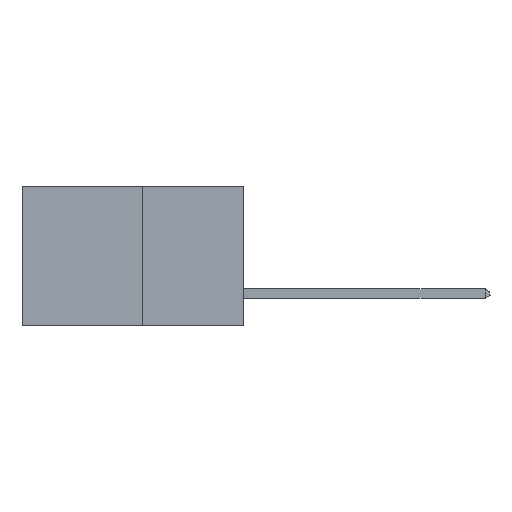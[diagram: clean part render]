
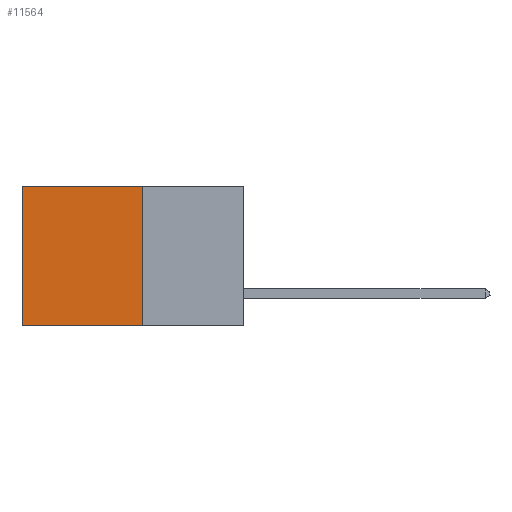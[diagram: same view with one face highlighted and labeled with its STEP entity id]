
A CAD part, left-side view. The second image highlights one B-rep face of the part: STEP entity #11564.
In plain terms, the highlighted planar face has unit normal (-1, 0, 0).
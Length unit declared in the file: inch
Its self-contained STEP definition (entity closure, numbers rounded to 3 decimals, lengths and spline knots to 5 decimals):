
#1414 = CARTESIAN_POINT ( 'NONE',  ( 0.277, 0.27, 0. ) ) ;
#2942 = DIRECTION ( 'NONE',  ( 0., 0., -1. ) ) ;
#2967 = CARTESIAN_POINT ( 'NONE',  ( 0.277, 0.27, -0.37 ) ) ;
#3269 = EDGE_CURVE ( 'NONE', #19605, #4331, #15075, .T. ) ;
#3989 = VECTOR ( 'NONE', #9598, 39.37008 ) ;
#4331 = VERTEX_POINT ( 'NONE', #9161 ) ;
#5077 = EDGE_LOOP ( 'NONE', ( #13645, #12473, #19442, #5239 ) ) ;
#5239 = ORIENTED_EDGE ( 'NONE', *, *, #6324, .T. ) ;
#5802 = VECTOR ( 'NONE', #19925, 39.37008 ) ;
#5838 = EDGE_CURVE ( 'NONE', #4331, #9906, #24892, .T. ) ;
#6324 = EDGE_CURVE ( 'NONE', #19605, #13140, #21268, .T. ) ;
#6867 = CARTESIAN_POINT ( 'NONE',  ( 0.277, 0.59, -0.37 ) ) ;
#7278 = CARTESIAN_POINT ( 'NONE',  ( 0.277, 0.27, -0.37 ) ) ;
#8807 = VECTOR ( 'NONE', #2942, 39.37008 ) ;
#9161 = CARTESIAN_POINT ( 'NONE',  ( 0.277, 0.27, -0.37 ) ) ;
#9311 = FACE_OUTER_BOUND ( 'NONE', #5077, .T. ) ;
#9427 = LINE ( 'NONE', #18610, #8807 ) ;
#9598 = DIRECTION ( 'NONE',  ( 0., 0., -1. ) ) ;
#9906 = VERTEX_POINT ( 'NONE', #6867 ) ;
#11564 = ADVANCED_FACE ( 'NONE', ( #9311 ), #13255, .F. ) ;
#11855 = AXIS2_PLACEMENT_3D ( 'NONE', #13756, #13218, #13209 ) ;
#12473 = ORIENTED_EDGE ( 'NONE', *, *, #5838, .F. ) ;
#13140 = VERTEX_POINT ( 'NONE', #23534 ) ;
#13209 = DIRECTION ( 'NONE',  ( 0., 0., -1. ) ) ;
#13218 = DIRECTION ( 'NONE',  ( 1., 0., 0. ) ) ;
#13255 = PLANE ( 'NONE',  #11855 ) ;
#13645 = ORIENTED_EDGE ( 'NONE', *, *, #24022, .T. ) ;
#13756 = CARTESIAN_POINT ( 'NONE',  ( 0.277, 0.27, -0.37 ) ) ;
#15075 = LINE ( 'NONE', #2967, #3989 ) ;
#15509 = VECTOR ( 'NONE', #21923, 39.37008 ) ;
#18610 = CARTESIAN_POINT ( 'NONE',  ( 0.277, 0.59, -0.37 ) ) ;
#19442 = ORIENTED_EDGE ( 'NONE', *, *, #3269, .F. ) ;
#19605 = VERTEX_POINT ( 'NONE', #1414 ) ;
#19925 = DIRECTION ( 'NONE',  ( 0., 1., 0. ) ) ;
#21268 = LINE ( 'NONE', #22076, #5802 ) ;
#21923 = DIRECTION ( 'NONE',  ( 0., 1., 0. ) ) ;
#22076 = CARTESIAN_POINT ( 'NONE',  ( 0.277, 0.27, 0. ) ) ;
#23534 = CARTESIAN_POINT ( 'NONE',  ( 0.277, 0.59, 0. ) ) ;
#24022 = EDGE_CURVE ( 'NONE', #13140, #9906, #9427, .T. ) ;
#24892 = LINE ( 'NONE', #7278, #15509 ) ;
